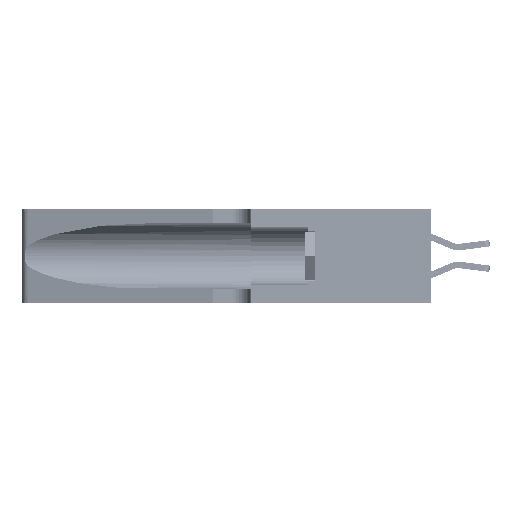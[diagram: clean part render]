
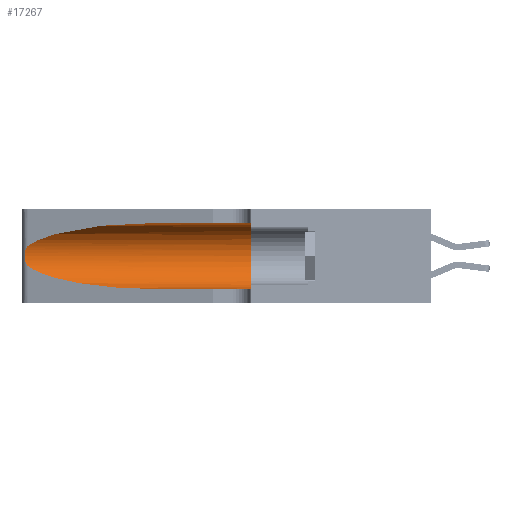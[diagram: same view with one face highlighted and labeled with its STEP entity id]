
A CAD part, left-side view. The second image highlights one B-rep face of the part: STEP entity #17267.
In plain terms, the highlighted cylindrical face has radius 3.308 mm (diameter 6.617 mm), a partial arc.
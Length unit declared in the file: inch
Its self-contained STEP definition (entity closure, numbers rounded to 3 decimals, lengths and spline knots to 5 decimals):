
#1082 = CIRCLE ( 'NONE', #44172, 0.13025 ) ;
#1247 = VERTEX_POINT ( 'NONE', #31461 ) ;
#2495 = CARTESIAN_POINT ( 'NONE',  ( 0.1305, 0.72297, 0.05475 ) ) ;
#2711 = CARTESIAN_POINT ( 'NONE',  ( 0.25487, 1.22718, 0.14631 ) ) ;
#2910 = DIRECTION ( 'NONE',  ( 0., -1., 0. ) ) ;
#2955 =( BOUNDED_CURVE ( )  B_SPLINE_CURVE ( 3, ( #30489, #5306, #13402, #8988 ),
 .UNSPECIFIED., .F., .F. ) 
 B_SPLINE_CURVE_WITH_KNOTS ( ( 4, 4 ),
 ( 1.5708, 2.84003 ),
 .UNSPECIFIED. ) 
 CURVE ( )  GEOMETRIC_REPRESENTATION_ITEM ( )  RATIONAL_B_SPLINE_CURVE ( ( 1., 0.87, 0.87, 1. ) ) 
 REPRESENTATION_ITEM ( '' )  );
#2997 = CARTESIAN_POINT ( 'NONE',  ( 0.25487, 1.22718, 0.22369 ) ) ;
#3085 = LINE ( 'NONE', #11410, #20158 ) ;
#3087 = CARTESIAN_POINT ( 'NONE',  ( 0.25555, 1.22993, 0.14849 ) ) ;
#3270 = CARTESIAN_POINT ( 'NONE',  ( 0.25789, 1.23486, 0.15765 ) ) ;
#4896 = CARTESIAN_POINT ( 'NONE',  ( 0.1305, 0.35, 0.05475 ) ) ;
#5286 = CARTESIAN_POINT ( 'NONE',  ( 0.25487, 1.22718, 0.14631 ) ) ;
#5306 = CARTESIAN_POINT ( 'NONE',  ( 0.18966, 0.96281, 0.31525 ) ) ;
#7103 = CARTESIAN_POINT ( 'NONE',  ( 0.25639, 1.23186, 0.15144 ) ) ;
#7323 = CARTESIAN_POINT ( 'NONE',  ( 0.1305, 0.35, 0.185 ) ) ;
#7517 = VERTEX_POINT ( 'NONE', #2495 ) ;
#7678 = CARTESIAN_POINT ( 'NONE',  ( 0.1305, 0.72297, 0.31525 ) ) ;
#8988 = CARTESIAN_POINT ( 'NONE',  ( 0.25487, 1.22718, 0.22369 ) ) ;
#10604 = VERTEX_POINT ( 'NONE', #2997 ) ;
#11410 = CARTESIAN_POINT ( 'NONE',  ( 0.1305, 1.61858, 0.05475 ) ) ;
#12775 = DIRECTION ( 'NONE',  ( 0., 0., -1. ) ) ;
#13263 = CYLINDRICAL_SURFACE ( 'NONE', #23038, 0.13025 ) ;
#13402 = CARTESIAN_POINT ( 'NONE',  ( 0.2373, 1.15595, 0.28018 ) ) ;
#13704 = CARTESIAN_POINT ( 'NONE',  ( 0.1305, 0.35, 0.31525 ) ) ;
#14116 = CARTESIAN_POINT ( 'NONE',  ( 0.2373, 1.15595, 0.08982 ) ) ;
#14337 = ORIENTED_EDGE ( 'NONE', *, *, #47203, .T. ) ;
#14505 = LINE ( 'NONE', #27708, #45454 ) ;
#15390 = B_SPLINE_CURVE_WITH_KNOTS ( 'NONE', 3,
 ( #48865, #23461, #45025, #53096, #19973, #52900, #31951, #15934, #27893, #48678, #3270, #7103, #3087, #2711 ),
 .UNSPECIFIED., .F., .F.,
 ( 4, 2, 2, 2, 2, 2, 4 ),
 ( 0., 0.00027, 0.00053, 0.00107, 0.0016, 0.00187, 0.00214 ),
 .UNSPECIFIED. ) ;
#15425 = DIRECTION ( 'NONE',  ( 0., 0., 1. ) ) ;
#15934 = CARTESIAN_POINT ( 'NONE',  ( 0.26075, 1.23896, 0.178 ) ) ;
#17267 = ADVANCED_FACE ( 'NONE', ( #38252 ), #13263, .F. ) ;
#19973 = CARTESIAN_POINT ( 'NONE',  ( 0.25854, 1.2359, 0.20912 ) ) ;
#20158 = VECTOR ( 'NONE', #28498, 39.37008 ) ;
#21641 = EDGE_CURVE ( 'NONE', #25790, #10604, #2955, .T. ) ;
#22725 = CARTESIAN_POINT ( 'NONE',  ( 0.1305, 0.72297, 0.05475 ) ) ;
#23038 = AXIS2_PLACEMENT_3D ( 'NONE', #34474, #33748, #12775 ) ;
#23461 = CARTESIAN_POINT ( 'NONE',  ( 0.25555, 1.22994, 0.2215 ) ) ;
#24296 = EDGE_CURVE ( 'NONE', #25790, #38270, #14505, .T. ) ;
#24301 = ORIENTED_EDGE ( 'NONE', *, *, #39675, .T. ) ;
#25790 = VERTEX_POINT ( 'NONE', #7678 ) ;
#26404 = CARTESIAN_POINT ( 'NONE',  ( 0.18966, 0.96281, 0.05475 ) ) ;
#27690 = EDGE_CURVE ( 'NONE', #38270, #41959, #1082, .T. ) ;
#27708 = CARTESIAN_POINT ( 'NONE',  ( 0.1305, 1.61858, 0.31525 ) ) ;
#27893 = CARTESIAN_POINT ( 'NONE',  ( 0.26017, 1.23833, 0.17102 ) ) ;
#28498 = DIRECTION ( 'NONE',  ( 0., -1., 0. ) ) ;
#30489 = CARTESIAN_POINT ( 'NONE',  ( 0.1305, 0.72297, 0.31525 ) ) ;
#30994 = ORIENTED_EDGE ( 'NONE', *, *, #27690, .F. ) ;
#31461 = CARTESIAN_POINT ( 'NONE',  ( 0.25487, 1.22718, 0.14631 ) ) ;
#31951 = CARTESIAN_POINT ( 'NONE',  ( 0.26075, 1.23896, 0.19203 ) ) ;
#33748 = DIRECTION ( 'NONE',  ( 0., -1., 0. ) ) ;
#34474 = CARTESIAN_POINT ( 'NONE',  ( 0.1305, 1.61858, 0.185 ) ) ;
#38252 = FACE_OUTER_BOUND ( 'NONE', #50093, .T. ) ;
#38270 = VERTEX_POINT ( 'NONE', #13704 ) ;
#39675 = EDGE_CURVE ( 'NONE', #1247, #7517, #54179, .T. ) ;
#41959 = VERTEX_POINT ( 'NONE', #4896 ) ;
#42950 = ORIENTED_EDGE ( 'NONE', *, *, #24296, .F. ) ;
#43882 = ORIENTED_EDGE ( 'NONE', *, *, #45619, .T. ) ;
#44172 = AXIS2_PLACEMENT_3D ( 'NONE', #7323, #44684, #15425 ) ;
#44684 = DIRECTION ( 'NONE',  ( 0., 1., 0. ) ) ;
#45025 = CARTESIAN_POINT ( 'NONE',  ( 0.25639, 1.23184, 0.21858 ) ) ;
#45454 = VECTOR ( 'NONE', #2910, 39.37008 ) ;
#45619 = EDGE_CURVE ( 'NONE', #10604, #1247, #15390, .T. ) ;
#47203 = EDGE_CURVE ( 'NONE', #7517, #41959, #3085, .T. ) ;
#48678 = CARTESIAN_POINT ( 'NONE',  ( 0.25856, 1.23593, 0.16098 ) ) ;
#48865 = CARTESIAN_POINT ( 'NONE',  ( 0.25487, 1.22718, 0.22369 ) ) ;
#50093 = EDGE_LOOP ( 'NONE', ( #52885, #43882, #24301, #14337, #30994, #42950 ) ) ;
#52885 = ORIENTED_EDGE ( 'NONE', *, *, #21641, .T. ) ;
#52900 = CARTESIAN_POINT ( 'NONE',  ( 0.26018, 1.23835, 0.19895 ) ) ;
#53096 = CARTESIAN_POINT ( 'NONE',  ( 0.25787, 1.23484, 0.2124 ) ) ;
#54179 =( BOUNDED_CURVE ( )  B_SPLINE_CURVE ( 3, ( #5286, #14116, #26404, #22725 ),
 .UNSPECIFIED., .F., .F. ) 
 B_SPLINE_CURVE_WITH_KNOTS ( ( 4, 4 ),
 ( 3.44316, 4.71239 ),
 .UNSPECIFIED. ) 
 CURVE ( )  GEOMETRIC_REPRESENTATION_ITEM ( )  RATIONAL_B_SPLINE_CURVE ( ( 1., 0.87, 0.87, 1. ) ) 
 REPRESENTATION_ITEM ( '' )  );
